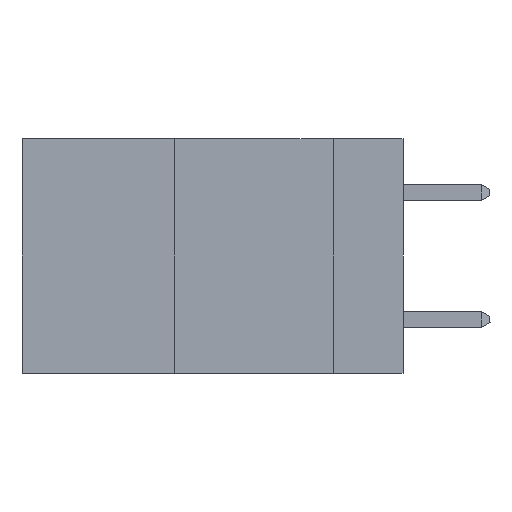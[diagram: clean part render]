
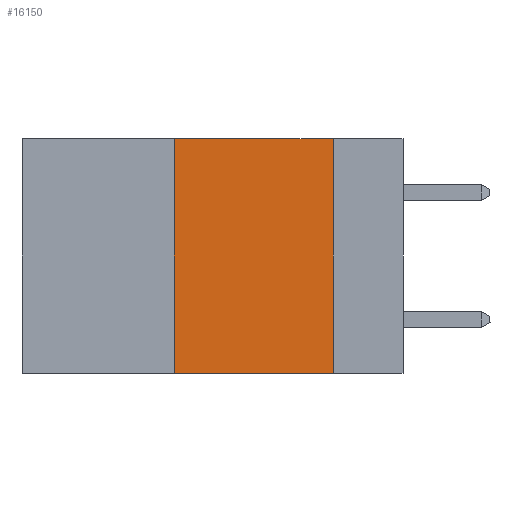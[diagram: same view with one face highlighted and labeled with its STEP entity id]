
A CAD part, left-side view. The second image highlights one B-rep face of the part: STEP entity #16150.
In plain terms, the highlighted planar face has unit normal (-1, 0, 0).
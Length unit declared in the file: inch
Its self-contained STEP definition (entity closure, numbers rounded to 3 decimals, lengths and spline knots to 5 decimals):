
#232 = ORIENTED_EDGE ( 'NONE', *, *, #4727, .F. ) ;
#450 = DIRECTION ( 'NONE',  ( 0., 0., -1. ) ) ;
#983 = EDGE_CURVE ( 'NONE', #13772, #15934, #9742, .T. ) ;
#2325 = CARTESIAN_POINT ( 'NONE',  ( 0., 0.6, 0. ) ) ;
#2456 = ORIENTED_EDGE ( 'NONE', *, *, #10754, .F. ) ;
#2712 = VECTOR ( 'NONE', #8507, 39.37008 ) ;
#3243 = AXIS2_PLACEMENT_3D ( 'NONE', #7219, #8487, #450 ) ;
#4107 = CARTESIAN_POINT ( 'NONE',  ( 0., 0.11, -0.37 ) ) ;
#4312 = EDGE_LOOP ( 'NONE', ( #232, #10077, #2456, #16582 ) ) ;
#4727 = EDGE_CURVE ( 'NONE', #14473, #15934, #15204, .T. ) ;
#5637 = CARTESIAN_POINT ( 'NONE',  ( 0., 0.11, 0. ) ) ;
#5723 = EDGE_CURVE ( 'NONE', #14437, #14473, #16738, .T. ) ;
#5903 = PLANE ( 'NONE',  #3243 ) ;
#7219 = CARTESIAN_POINT ( 'NONE',  ( 0., 0.6, 0. ) ) ;
#8487 = DIRECTION ( 'NONE',  ( 1., 0., 0. ) ) ;
#8507 = DIRECTION ( 'NONE',  ( 0., -1., 0. ) ) ;
#8898 = VECTOR ( 'NONE', #11145, 39.37008 ) ;
#9451 = CARTESIAN_POINT ( 'NONE',  ( 0., 0.36, -0.37 ) ) ;
#9487 = CARTESIAN_POINT ( 'NONE',  ( 0., 0.36, 0. ) ) ;
#9742 = LINE ( 'NONE', #11065, #2712 ) ;
#10077 = ORIENTED_EDGE ( 'NONE', *, *, #5723, .F. ) ;
#10754 = EDGE_CURVE ( 'NONE', #13772, #14437, #12260, .T. ) ;
#11065 = CARTESIAN_POINT ( 'NONE',  ( 0., 0.6, -0.37 ) ) ;
#11145 = DIRECTION ( 'NONE',  ( 0., 0., 1. ) ) ;
#11858 = VECTOR ( 'NONE', #14596, 39.37008 ) ;
#12260 = LINE ( 'NONE', #13621, #8898 ) ;
#12513 = DIRECTION ( 'NONE',  ( 0., -1., 0. ) ) ;
#13408 = VECTOR ( 'NONE', #12513, 39.37008 ) ;
#13621 = CARTESIAN_POINT ( 'NONE',  ( 0., 0.36, 0. ) ) ;
#13772 = VERTEX_POINT ( 'NONE', #9451 ) ;
#14437 = VERTEX_POINT ( 'NONE', #9487 ) ;
#14473 = VERTEX_POINT ( 'NONE', #5637 ) ;
#14551 = FACE_OUTER_BOUND ( 'NONE', #4312, .T. ) ;
#14596 = DIRECTION ( 'NONE',  ( 0., 0., -1. ) ) ;
#15204 = LINE ( 'NONE', #15762, #11858 ) ;
#15762 = CARTESIAN_POINT ( 'NONE',  ( 0., 0.11, 0. ) ) ;
#15934 = VERTEX_POINT ( 'NONE', #4107 ) ;
#16150 = ADVANCED_FACE ( 'NONE', ( #14551 ), #5903, .F. ) ;
#16582 = ORIENTED_EDGE ( 'NONE', *, *, #983, .T. ) ;
#16738 = LINE ( 'NONE', #2325, #13408 ) ;
